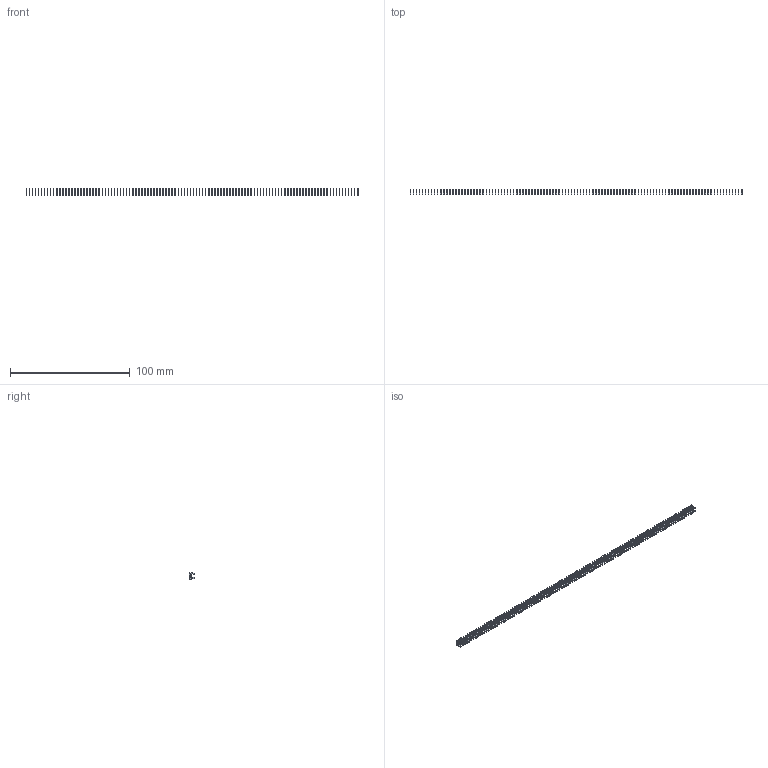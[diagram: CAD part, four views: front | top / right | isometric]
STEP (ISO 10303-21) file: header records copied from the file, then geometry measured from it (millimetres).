
FILE_DESCRIPTION (( 'STEP AP203' ), '1' );
FILE_NAME ('105-110-208-100.STEP', '2020-04-08T01:22:42', ( '' ), ( '' ), 'SwSTEP 2.0', 'SolidWorks 2016', '' );
FILE_SCHEMA (( 'CONFIG_CONTROL_DESIGN' ));
Length unit declared in the file: inch
Products named in the file (2): 105-110-208-100; 100-290-001_100-290-208
Assembly tree (110 placements, depth 2):
  105-110-208-100
    100-290-001_100-290-208  x110
Bounding box: 277.37 x 4.82 x 5.17 mm (x, y, z)
Volume: 756.9 mm3; surface area: 4674.6 mm2
Topology: 110 solids, 110 shells, 2750 faces, 7590 edges, 5060 vertices
Faces by surface type: plane 2420, cylinder 330
Entity records: 4477 total; most frequent: DIRECTION 351, CARTESIAN_POINT 253, COORDINATED_UNIVERSAL_TIME_OFFSET 230, CALENDAR_DATE 230, DATE_AND_TIME 230, LOCAL_TIME 230, AXIS2_PLACEMENT_3D 144, ORIENTED_EDGE 138
